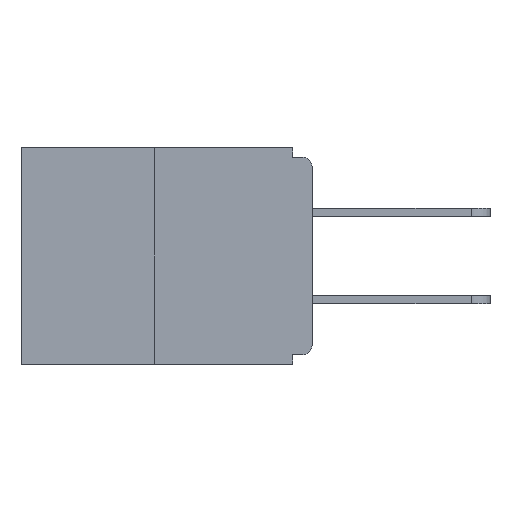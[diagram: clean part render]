
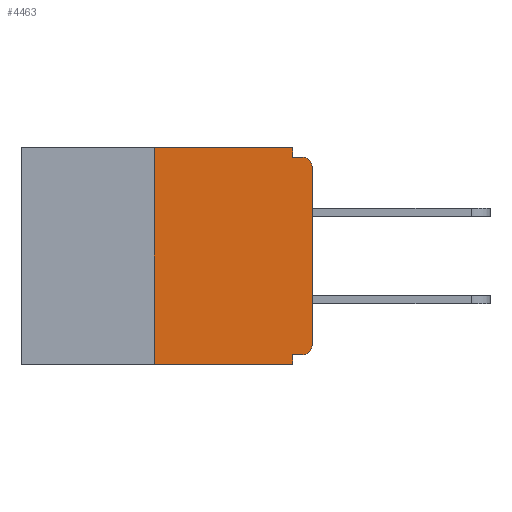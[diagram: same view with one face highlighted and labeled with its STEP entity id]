
A CAD part, left-side view. The second image highlights one B-rep face of the part: STEP entity #4463.
In plain terms, the highlighted planar face has unit normal (-1, 0, 0).
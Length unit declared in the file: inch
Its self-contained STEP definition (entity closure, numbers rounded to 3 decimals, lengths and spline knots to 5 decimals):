
#6 = ORIENTED_EDGE ( 'NONE', *, *, #1500, .T. ) ;
#361 = ORIENTED_EDGE ( 'NONE', *, *, #3374, .T. ) ;
#370 = EDGE_LOOP ( 'NONE', ( #6705, #6440, #361, #10995, #10947, #5294, #6, #5836, #3357, #10456 ) ) ;
#687 = EDGE_CURVE ( 'NONE', #6201, #7369, #1678, .T. ) ;
#960 = VECTOR ( 'NONE', #8782, 39.37008 ) ;
#1246 = VECTOR ( 'NONE', #6290, 39.37008 ) ;
#1364 = CARTESIAN_POINT ( 'NONE',  ( 0., 0.031, -0.343 ) ) ;
#1497 = VECTOR ( 'NONE', #11128, 39.37008 ) ;
#1500 = EDGE_CURVE ( 'NONE', #2016, #8162, #8733, .T. ) ;
#1678 = LINE ( 'NONE', #7809, #9198 ) ;
#1716 = CARTESIAN_POINT ( 'NONE',  ( 0., 0.031, -0.328 ) ) ;
#1724 = CARTESIAN_POINT ( 'NONE',  ( 0., 0.015, -0.313 ) ) ;
#2016 = VERTEX_POINT ( 'NONE', #7700 ) ;
#2050 = DIRECTION ( 'NONE',  ( -1., 0., 0. ) ) ;
#2468 = LINE ( 'NONE', #4177, #1497 ) ;
#2485 = DIRECTION ( 'NONE',  ( 0., -1., 0. ) ) ;
#2717 = CARTESIAN_POINT ( 'NONE',  ( 0., 0.25, 0. ) ) ;
#3008 = CARTESIAN_POINT ( 'NONE',  ( 0., 0.46, -0.343 ) ) ;
#3067 = VERTEX_POINT ( 'NONE', #7172 ) ;
#3129 = CARTESIAN_POINT ( 'NONE',  ( 0., 0., -0.03 ) ) ;
#3213 = CARTESIAN_POINT ( 'NONE',  ( 0., 0.015, -0.015 ) ) ;
#3345 = LINE ( 'NONE', #10337, #5929 ) ;
#3357 = ORIENTED_EDGE ( 'NONE', *, *, #687, .F. ) ;
#3374 = EDGE_CURVE ( 'NONE', #5352, #7729, #4133, .T. ) ;
#3471 = CARTESIAN_POINT ( 'NONE',  ( 0., 0., 0. ) ) ;
#3758 = CIRCLE ( 'NONE', #10164, 0.015 ) ;
#3851 = FACE_OUTER_BOUND ( 'NONE', #370, .T. ) ;
#3879 = EDGE_CURVE ( 'NONE', #10876, #3067, #6973, .T. ) ;
#4133 = LINE ( 'NONE', #3008, #6736 ) ;
#4177 = CARTESIAN_POINT ( 'NONE',  ( 0., 0., -0.328 ) ) ;
#4463 = ADVANCED_FACE ( 'NONE', ( #3851 ), #5414, .F. ) ;
#4615 = CARTESIAN_POINT ( 'NONE',  ( 0., 0.031, 0. ) ) ;
#4647 = DIRECTION ( 'NONE',  ( 0., 0., -1. ) ) ;
#4715 = EDGE_CURVE ( 'NONE', #9751, #7729, #3345, .T. ) ;
#4826 = EDGE_CURVE ( 'NONE', #5352, #10876, #10613, .T. ) ;
#5294 = ORIENTED_EDGE ( 'NONE', *, *, #5409, .T. ) ;
#5302 = DIRECTION ( 'NONE',  ( 0., -1., 0. ) ) ;
#5352 = VERTEX_POINT ( 'NONE', #9273 ) ;
#5409 = EDGE_CURVE ( 'NONE', #6609, #2016, #6848, .T. ) ;
#5414 = PLANE ( 'NONE',  #6831 ) ;
#5566 = AXIS2_PLACEMENT_3D ( 'NONE', #1724, #7038, #9670 ) ;
#5836 = ORIENTED_EDGE ( 'NONE', *, *, #11195, .T. ) ;
#5929 = VECTOR ( 'NONE', #8718, 39.37008 ) ;
#6032 = CARTESIAN_POINT ( 'NONE',  ( 0., 0.031, -0.015 ) ) ;
#6201 = VERTEX_POINT ( 'NONE', #6032 ) ;
#6290 = DIRECTION ( 'NONE',  ( 0., 0., -1. ) ) ;
#6296 = VECTOR ( 'NONE', #10781, 39.37008 ) ;
#6440 = ORIENTED_EDGE ( 'NONE', *, *, #4826, .F. ) ;
#6588 = EDGE_CURVE ( 'NONE', #6609, #9751, #2468, .T. ) ;
#6609 = VERTEX_POINT ( 'NONE', #9333 ) ;
#6705 = ORIENTED_EDGE ( 'NONE', *, *, #3879, .F. ) ;
#6736 = VECTOR ( 'NONE', #9995, 39.37008 ) ;
#6831 = AXIS2_PLACEMENT_3D ( 'NONE', #7346, #7176, #4647 ) ;
#6848 = CIRCLE ( 'NONE', #5566, 0.015 ) ;
#6973 = LINE ( 'NONE', #10473, #8384 ) ;
#7038 = DIRECTION ( 'NONE',  ( -1., 0., 0. ) ) ;
#7144 = CARTESIAN_POINT ( 'NONE',  ( 0., 0.015, -0.03 ) ) ;
#7172 = CARTESIAN_POINT ( 'NONE',  ( 0., 0.031, 0. ) ) ;
#7176 = DIRECTION ( 'NONE',  ( 1., 0., 0. ) ) ;
#7346 = CARTESIAN_POINT ( 'NONE',  ( 0., 0.46, 0. ) ) ;
#7369 = VERTEX_POINT ( 'NONE', #3213 ) ;
#7700 = CARTESIAN_POINT ( 'NONE',  ( 0., 0., -0.313 ) ) ;
#7729 = VERTEX_POINT ( 'NONE', #1364 ) ;
#7809 = CARTESIAN_POINT ( 'NONE',  ( 0., 0., -0.015 ) ) ;
#8113 = LINE ( 'NONE', #4615, #1246 ) ;
#8162 = VERTEX_POINT ( 'NONE', #3129 ) ;
#8384 = VECTOR ( 'NONE', #5302, 39.37008 ) ;
#8718 = DIRECTION ( 'NONE',  ( 0., 0., -1. ) ) ;
#8733 = LINE ( 'NONE', #3471, #960 ) ;
#8782 = DIRECTION ( 'NONE',  ( 0., 0., 1. ) ) ;
#9198 = VECTOR ( 'NONE', #2485, 39.37008 ) ;
#9273 = CARTESIAN_POINT ( 'NONE',  ( 0., 0.25, -0.343 ) ) ;
#9333 = CARTESIAN_POINT ( 'NONE',  ( 0., 0.015, -0.328 ) ) ;
#9670 = DIRECTION ( 'NONE',  ( 0., 0., -1. ) ) ;
#9688 = CARTESIAN_POINT ( 'NONE',  ( 0., 0.25, 0. ) ) ;
#9751 = VERTEX_POINT ( 'NONE', #1716 ) ;
#9892 = DIRECTION ( 'NONE',  ( 0., 0., -1. ) ) ;
#9995 = DIRECTION ( 'NONE',  ( 0., -1., 0. ) ) ;
#10164 = AXIS2_PLACEMENT_3D ( 'NONE', #7144, #2050, #9892 ) ;
#10337 = CARTESIAN_POINT ( 'NONE',  ( 0., 0.031, -0.343 ) ) ;
#10456 = ORIENTED_EDGE ( 'NONE', *, *, #11182, .F. ) ;
#10473 = CARTESIAN_POINT ( 'NONE',  ( 0., 0.46, 0. ) ) ;
#10613 = LINE ( 'NONE', #9688, #6296 ) ;
#10781 = DIRECTION ( 'NONE',  ( 0., 0., 1. ) ) ;
#10876 = VERTEX_POINT ( 'NONE', #2717 ) ;
#10947 = ORIENTED_EDGE ( 'NONE', *, *, #6588, .F. ) ;
#10995 = ORIENTED_EDGE ( 'NONE', *, *, #4715, .F. ) ;
#11128 = DIRECTION ( 'NONE',  ( 0., 1., 0. ) ) ;
#11182 = EDGE_CURVE ( 'NONE', #3067, #6201, #8113, .T. ) ;
#11195 = EDGE_CURVE ( 'NONE', #8162, #7369, #3758, .T. ) ;
